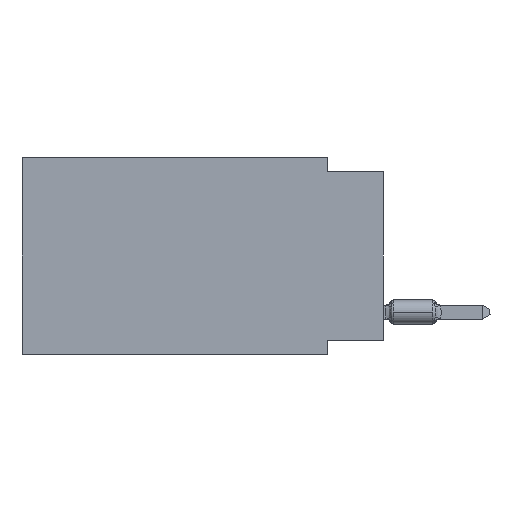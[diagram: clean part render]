
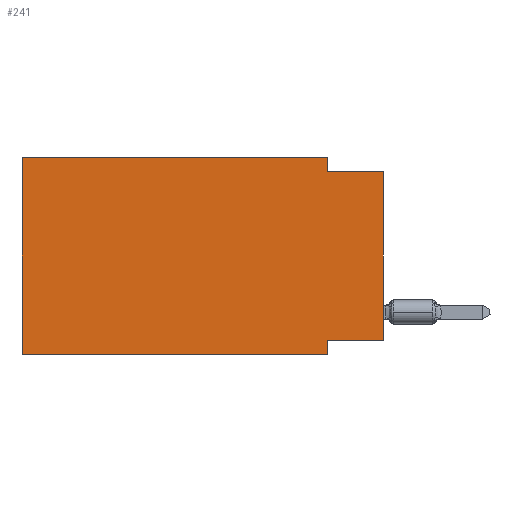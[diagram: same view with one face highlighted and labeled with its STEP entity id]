
A CAD part, left-side view. The second image highlights one B-rep face of the part: STEP entity #241.
In plain terms, the highlighted planar face has unit normal (-1, 0, 0).
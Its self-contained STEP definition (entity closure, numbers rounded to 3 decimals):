
#241 = ADVANCED_FACE ( 'NONE', ( #69944 ), #10336, .F. ) ;
#2503 = ORIENTED_EDGE ( 'NONE', *, *, #4948, .F. ) ;
#2789 = CARTESIAN_POINT ( 'NONE',  ( 0., 16.383, -8.89 ) ) ;
#4298 = DIRECTION ( 'NONE',  ( 0., 0., -1. ) ) ;
#4948 = EDGE_CURVE ( 'NONE', #14220, #58889, #5849, .T. ) ;
#5118 = CARTESIAN_POINT ( 'NONE',  ( 0., 2.54, 0. ) ) ;
#5301 = CARTESIAN_POINT ( 'NONE',  ( 0., 0., 0. ) ) ;
#5481 = AXIS2_PLACEMENT_3D ( 'NONE', #10753, #63843, #83842 ) ;
#5849 = LINE ( 'NONE', #57253, #36544 ) ;
#9388 = ORIENTED_EDGE ( 'NONE', *, *, #73307, .F. ) ;
#10336 = PLANE ( 'NONE',  #5481 ) ;
#10753 = CARTESIAN_POINT ( 'NONE',  ( 0., 16.383, 0. ) ) ;
#11630 = VECTOR ( 'NONE', #4298, 1000. ) ;
#11847 = DIRECTION ( 'NONE',  ( 0., 0., 1. ) ) ;
#12522 = CARTESIAN_POINT ( 'NONE',  ( 0., 16.383, 0. ) ) ;
#13696 = EDGE_CURVE ( 'NONE', #16522, #58889, #80102, .T. ) ;
#14220 = VERTEX_POINT ( 'NONE', #53066 ) ;
#14953 = VECTOR ( 'NONE', #49799, 1000. ) ;
#15838 = CARTESIAN_POINT ( 'NONE',  ( 0., 0., -0.635 ) ) ;
#15953 = EDGE_CURVE ( 'NONE', #68204, #65599, #27175, .T. ) ;
#16522 = VERTEX_POINT ( 'NONE', #54477 ) ;
#19059 = CARTESIAN_POINT ( 'NONE',  ( 0., 2.54, -8.89 ) ) ;
#19311 = ORIENTED_EDGE ( 'NONE', *, *, #13696, .T. ) ;
#20329 = VECTOR ( 'NONE', #54574, 1000. ) ;
#22981 = ORIENTED_EDGE ( 'NONE', *, *, #66090, .F. ) ;
#23449 = VECTOR ( 'NONE', #38819, 1000. ) ;
#24839 = CARTESIAN_POINT ( 'NONE',  ( 0., 2.54, 0. ) ) ;
#27091 = EDGE_CURVE ( 'NONE', #57182, #65556, #72155, .T. ) ;
#27175 = LINE ( 'NONE', #66323, #20329 ) ;
#28995 = LINE ( 'NONE', #62057, #54204 ) ;
#31255 = CARTESIAN_POINT ( 'NONE',  ( 0., 2.54, -8.89 ) ) ;
#34715 = ORIENTED_EDGE ( 'NONE', *, *, #27091, .F. ) ;
#35391 = VECTOR ( 'NONE', #11847, 1000. ) ;
#36328 = LINE ( 'NONE', #61568, #14953 ) ;
#36544 = VECTOR ( 'NONE', #78532, 1000. ) ;
#37362 = VECTOR ( 'NONE', #78766, 1000. ) ;
#38819 = DIRECTION ( 'NONE',  ( 0., 0., 1. ) ) ;
#39932 = CARTESIAN_POINT ( 'NONE',  ( 0., 2.54, -8.255 ) ) ;
#42801 = EDGE_CURVE ( 'NONE', #65599, #14220, #59201, .T. ) ;
#49799 = DIRECTION ( 'NONE',  ( 0., -1., 0. ) ) ;
#52164 = EDGE_LOOP ( 'NONE', ( #19311, #2503, #73181, #80654, #22981, #66402, #34715, #9388 ) ) ;
#53066 = CARTESIAN_POINT ( 'NONE',  ( 0., 2.54, -0.635 ) ) ;
#54204 = VECTOR ( 'NONE', #82051, 1000. ) ;
#54477 = CARTESIAN_POINT ( 'NONE',  ( 0., 0., -8.255 ) ) ;
#54574 = DIRECTION ( 'NONE',  ( 0., -1., 0. ) ) ;
#55001 = VERTEX_POINT ( 'NONE', #2789 ) ;
#57182 = VERTEX_POINT ( 'NONE', #39932 ) ;
#57253 = CARTESIAN_POINT ( 'NONE',  ( 0., 0., -0.635 ) ) ;
#58848 = CARTESIAN_POINT ( 'NONE',  ( 0., 16.383, 0. ) ) ;
#58889 = VERTEX_POINT ( 'NONE', #15838 ) ;
#59201 = LINE ( 'NONE', #24839, #37362 ) ;
#61568 = CARTESIAN_POINT ( 'NONE',  ( 0., 16.383, -8.89 ) ) ;
#62057 = CARTESIAN_POINT ( 'NONE',  ( 0., 0., -8.255 ) ) ;
#63843 = DIRECTION ( 'NONE',  ( 1., 0., 0. ) ) ;
#64790 = EDGE_CURVE ( 'NONE', #55001, #65556, #36328, .T. ) ;
#65556 = VERTEX_POINT ( 'NONE', #31255 ) ;
#65599 = VERTEX_POINT ( 'NONE', #5118 ) ;
#66090 = EDGE_CURVE ( 'NONE', #55001, #68204, #84940, .T. ) ;
#66323 = CARTESIAN_POINT ( 'NONE',  ( 0., 16.383, 0. ) ) ;
#66402 = ORIENTED_EDGE ( 'NONE', *, *, #64790, .T. ) ;
#68204 = VERTEX_POINT ( 'NONE', #12522 ) ;
#69944 = FACE_OUTER_BOUND ( 'NONE', #52164, .T. ) ;
#72155 = LINE ( 'NONE', #19059, #11630 ) ;
#73181 = ORIENTED_EDGE ( 'NONE', *, *, #42801, .F. ) ;
#73307 = EDGE_CURVE ( 'NONE', #16522, #57182, #28995, .T. ) ;
#78532 = DIRECTION ( 'NONE',  ( 0., -1., 0. ) ) ;
#78766 = DIRECTION ( 'NONE',  ( 0., 0., -1. ) ) ;
#80102 = LINE ( 'NONE', #5301, #35391 ) ;
#80654 = ORIENTED_EDGE ( 'NONE', *, *, #15953, .F. ) ;
#82051 = DIRECTION ( 'NONE',  ( 0., 1., 0. ) ) ;
#83842 = DIRECTION ( 'NONE',  ( 0., 0., -1. ) ) ;
#84940 = LINE ( 'NONE', #58848, #23449 ) ;
